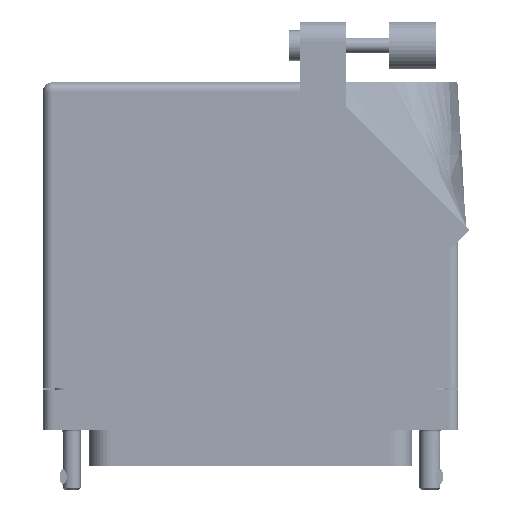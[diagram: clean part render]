
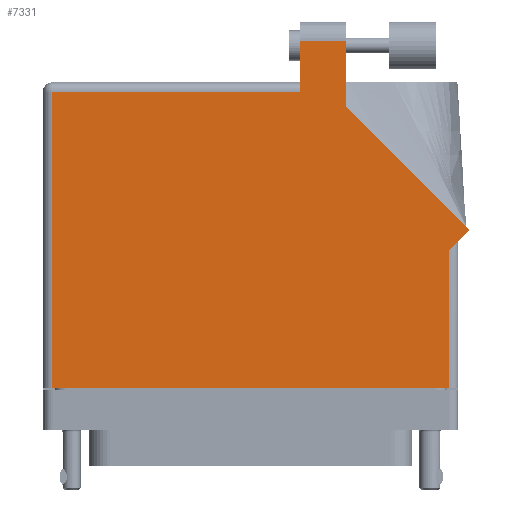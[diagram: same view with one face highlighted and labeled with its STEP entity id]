
A CAD part, front view. The second image highlights one B-rep face of the part: STEP entity #7331.
In plain terms, the highlighted face is planar.
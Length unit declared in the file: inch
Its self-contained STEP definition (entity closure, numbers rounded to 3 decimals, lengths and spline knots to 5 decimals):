
#2809 = CARTESIAN_POINT ( 'NONE',  ( 0.6345, 1.76442, 0.765 ) ) ;
#3124 = VECTOR ( 'NONE', #14938, 39.37008 ) ;
#3663 = VECTOR ( 'NONE', #51651, 39.37008 ) ;
#3768 = CARTESIAN_POINT ( 'NONE',  ( -1.3155, -0.1, 0.765 ) ) ;
#6549 = DIRECTION ( 'NONE',  ( -1., 0., 0. ) ) ;
#7331 = ADVANCED_FACE ( 'NONE', ( #23515 ), #93734, .F. ) ;
#8007 = LINE ( 'NONE', #3768, #10507 ) ;
#9378 = CARTESIAN_POINT ( 'NONE',  ( 1.3155, 0.88, 0.765 ) ) ;
#10507 = VECTOR ( 'NONE', #90305, 39.37008 ) ;
#10564 = CARTESIAN_POINT ( 'NONE',  ( 0.3275, 1.868, 0.765 ) ) ;
#13687 = EDGE_LOOP ( 'NONE', ( #99569, #34493, #60129, #84291, #17091, #53691, #50426, #88147, #71799 ) ) ;
#14938 = DIRECTION ( 'NONE',  ( 0., -1., 0. ) ) ;
#15898 = VECTOR ( 'NONE', #66761, 39.37008 ) ;
#16596 = EDGE_CURVE ( 'NONE', #65029, #49601, #8007, .T. ) ;
#17091 = ORIENTED_EDGE ( 'NONE', *, *, #16596, .T. ) ;
#18123 = LINE ( 'NONE', #96519, #29306 ) ;
#19474 = CARTESIAN_POINT ( 'NONE',  ( 0.3275, 2.205, 0.765 ) ) ;
#19665 = CARTESIAN_POINT ( 'NONE',  ( 1.44821, 0.95071, 0.765 ) ) ;
#19978 = EDGE_CURVE ( 'NONE', #72696, #71215, #77875, .T. ) ;
#23515 = FACE_OUTER_BOUND ( 'NONE', #13687, .T. ) ;
#29306 = VECTOR ( 'NONE', #32285, 39.37008 ) ;
#30421 = CARTESIAN_POINT ( 'NONE',  ( 1.44821, 0.95071, 0.765 ) ) ;
#30576 = CARTESIAN_POINT ( 'NONE',  ( 0.3275, 1.93, 0.765 ) ) ;
#30801 = VECTOR ( 'NONE', #94136, 39.37008 ) ;
#32285 = DIRECTION ( 'NONE',  ( -1., 0., 0. ) ) ;
#34493 = ORIENTED_EDGE ( 'NONE', *, *, #62108, .T. ) ;
#34921 = LINE ( 'NONE', #82327, #90878 ) ;
#39899 = VERTEX_POINT ( 'NONE', #87023 ) ;
#39916 = CARTESIAN_POINT ( 'NONE',  ( 1.3775, 0.88, 0.765 ) ) ;
#42034 = LINE ( 'NONE', #19474, #15898 ) ;
#42916 = LINE ( 'NONE', #30576, #3124 ) ;
#49601 = VERTEX_POINT ( 'NONE', #70690 ) ;
#50426 = ORIENTED_EDGE ( 'NONE', *, *, #19978, .T. ) ;
#51025 = VERTEX_POINT ( 'NONE', #65985 ) ;
#51432 = DIRECTION ( 'NONE',  ( 0., 1., 0. ) ) ;
#51651 = DIRECTION ( 'NONE',  ( -0.707, 0.707, 0. ) ) ;
#52945 = EDGE_CURVE ( 'NONE', #54893, #51025, #78217, .T. ) ;
#53681 = CARTESIAN_POINT ( 'NONE',  ( -1.3155, 1.868, 0.765 ) ) ;
#53691 = ORIENTED_EDGE ( 'NONE', *, *, #78418, .T. ) ;
#54116 = DIRECTION ( 'NONE',  ( 0., 0., -1. ) ) ;
#54893 = VERTEX_POINT ( 'NONE', #30421 ) ;
#56586 = AXIS2_PLACEMENT_3D ( 'NONE', #101723, #54116, #6549 ) ;
#56742 = VECTOR ( 'NONE', #64996, 39.37008 ) ;
#58331 = DIRECTION ( 'NONE',  ( 1., 0., 0. ) ) ;
#60039 = EDGE_CURVE ( 'NONE', #51025, #66018, #100973, .T. ) ;
#60129 = ORIENTED_EDGE ( 'NONE', *, *, #101115, .T. ) ;
#62108 = EDGE_CURVE ( 'NONE', #66018, #39899, #42034, .T. ) ;
#64996 = DIRECTION ( 'NONE',  ( 0., 1., 0. ) ) ;
#65029 = VERTEX_POINT ( 'NONE', #53681 ) ;
#65472 = VERTEX_POINT ( 'NONE', #10564 ) ;
#65985 = CARTESIAN_POINT ( 'NONE',  ( 0.6345, 1.76442, 0.765 ) ) ;
#66018 = VERTEX_POINT ( 'NONE', #99022 ) ;
#66761 = DIRECTION ( 'NONE',  ( -1., 0., 0. ) ) ;
#70690 = CARTESIAN_POINT ( 'NONE',  ( -1.3155, -0.1, 0.765 ) ) ;
#71215 = VERTEX_POINT ( 'NONE', #80128 ) ;
#71799 = ORIENTED_EDGE ( 'NONE', *, *, #52945, .T. ) ;
#72696 = VERTEX_POINT ( 'NONE', #79369 ) ;
#77875 = LINE ( 'NONE', #9378, #56742 ) ;
#78217 = LINE ( 'NONE', #19665, #3663 ) ;
#78418 = EDGE_CURVE ( 'NONE', #49601, #72696, #34921, .T. ) ;
#79369 = CARTESIAN_POINT ( 'NONE',  ( 1.3155, -0.1, 0.765 ) ) ;
#80128 = CARTESIAN_POINT ( 'NONE',  ( 1.3155, 0.818, 0.765 ) ) ;
#82327 = CARTESIAN_POINT ( 'NONE',  ( -1.3775, -0.1, 0.765 ) ) ;
#84291 = ORIENTED_EDGE ( 'NONE', *, *, #84702, .T. ) ;
#84702 = EDGE_CURVE ( 'NONE', #65472, #65029, #18123, .T. ) ;
#87023 = CARTESIAN_POINT ( 'NONE',  ( 0.3275, 2.205, 0.765 ) ) ;
#88147 = ORIENTED_EDGE ( 'NONE', *, *, #99463, .T. ) ;
#90305 = DIRECTION ( 'NONE',  ( 0., -1., 0. ) ) ;
#90878 = VECTOR ( 'NONE', #58331, 39.37008 ) ;
#93734 = PLANE ( 'NONE',  #56586 ) ;
#94136 = DIRECTION ( 'NONE',  ( 0.707, 0.707, 0. ) ) ;
#96519 = CARTESIAN_POINT ( 'NONE',  ( -1.3775, 1.868, 0.765 ) ) ;
#97076 = VECTOR ( 'NONE', #51432, 39.37008 ) ;
#99022 = CARTESIAN_POINT ( 'NONE',  ( 0.6345, 2.205, 0.765 ) ) ;
#99218 = LINE ( 'NONE', #39916, #30801 ) ;
#99463 = EDGE_CURVE ( 'NONE', #71215, #54893, #99218, .T. ) ;
#99569 = ORIENTED_EDGE ( 'NONE', *, *, #60039, .T. ) ;
#100973 = LINE ( 'NONE', #2809, #97076 ) ;
#101115 = EDGE_CURVE ( 'NONE', #39899, #65472, #42916, .T. ) ;
#101723 = CARTESIAN_POINT ( 'NONE',  ( -1.3775, 1.93, 0.765 ) ) ;
